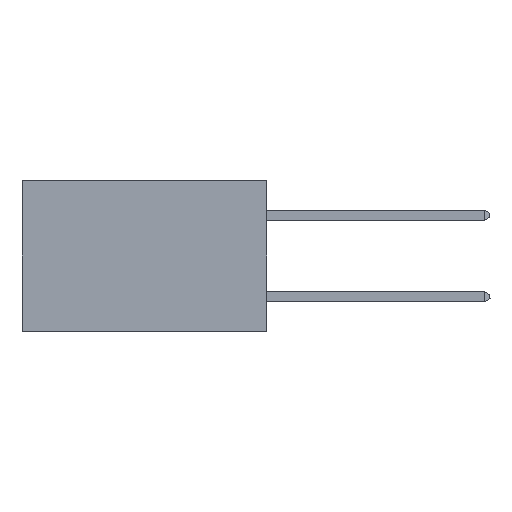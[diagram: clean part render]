
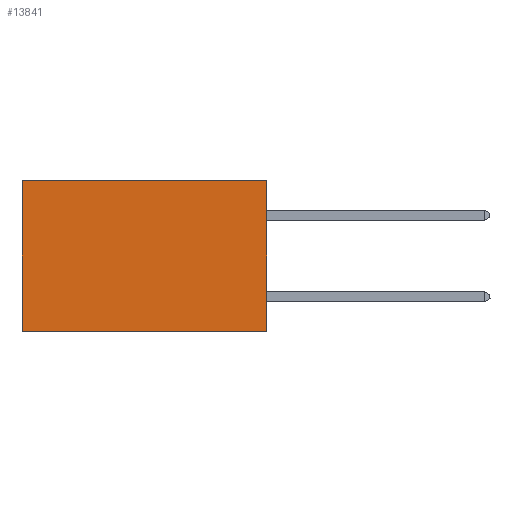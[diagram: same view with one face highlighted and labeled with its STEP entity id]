
A CAD part, left-side view. The second image highlights one B-rep face of the part: STEP entity #13841.
In plain terms, the highlighted planar face has unit normal (-1, 0, 0).
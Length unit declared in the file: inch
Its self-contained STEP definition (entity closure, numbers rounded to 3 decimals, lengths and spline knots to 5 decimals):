
#103 = DIRECTION ( 'NONE',  ( 1., 0., 0. ) ) ;
#491 = VERTEX_POINT ( 'NONE', #4262 ) ;
#1668 = EDGE_CURVE ( 'NONE', #12954, #12230, #16529, .T. ) ;
#2111 = DIRECTION ( 'NONE',  ( 0., 0., -1. ) ) ;
#2417 = EDGE_CURVE ( 'NONE', #12954, #491, #9904, .T. ) ;
#3598 = AXIS2_PLACEMENT_3D ( 'NONE', #10663, #103, #8134 ) ;
#4032 = DIRECTION ( 'NONE',  ( 0., 1., 0. ) ) ;
#4103 = ORIENTED_EDGE ( 'NONE', *, *, #1668, .T. ) ;
#4262 = CARTESIAN_POINT ( 'NONE',  ( 0.2875, 0., -0.37 ) ) ;
#4274 = CARTESIAN_POINT ( 'NONE',  ( 0.2875, 0., 0. ) ) ;
#6805 = PLANE ( 'NONE',  #3598 ) ;
#7149 = VERTEX_POINT ( 'NONE', #11163 ) ;
#7291 = EDGE_CURVE ( 'NONE', #491, #7149, #14238, .T. ) ;
#7792 = CARTESIAN_POINT ( 'NONE',  ( 0.2875, 0., 0. ) ) ;
#8134 = DIRECTION ( 'NONE',  ( 0., 0., -1. ) ) ;
#8281 = EDGE_LOOP ( 'NONE', ( #15273, #16694, #11215, #4103 ) ) ;
#9147 = CARTESIAN_POINT ( 'NONE',  ( 0.2875, 0., 0. ) ) ;
#9434 = DIRECTION ( 'NONE',  ( 0., 0., -1. ) ) ;
#9902 = VECTOR ( 'NONE', #4032, 39.37008 ) ;
#9904 = LINE ( 'NONE', #4274, #15490 ) ;
#10663 = CARTESIAN_POINT ( 'NONE',  ( 0.2875, 0., 0. ) ) ;
#11163 = CARTESIAN_POINT ( 'NONE',  ( 0.2875, 0.6, -0.37 ) ) ;
#11215 = ORIENTED_EDGE ( 'NONE', *, *, #2417, .F. ) ;
#12230 = VERTEX_POINT ( 'NONE', #16249 ) ;
#12257 = CARTESIAN_POINT ( 'NONE',  ( 0.2875, 0., -0.37 ) ) ;
#12954 = VERTEX_POINT ( 'NONE', #9147 ) ;
#13289 = DIRECTION ( 'NONE',  ( 0., 1., 0. ) ) ;
#13841 = ADVANCED_FACE ( 'NONE', ( #15282 ), #6805, .F. ) ;
#13993 = CARTESIAN_POINT ( 'NONE',  ( 0.2875, 0.6, 0. ) ) ;
#14238 = LINE ( 'NONE', #12257, #16549 ) ;
#14711 = EDGE_CURVE ( 'NONE', #12230, #7149, #16672, .T. ) ;
#14991 = VECTOR ( 'NONE', #2111, 39.37008 ) ;
#15273 = ORIENTED_EDGE ( 'NONE', *, *, #14711, .T. ) ;
#15282 = FACE_OUTER_BOUND ( 'NONE', #8281, .T. ) ;
#15490 = VECTOR ( 'NONE', #9434, 39.37008 ) ;
#16249 = CARTESIAN_POINT ( 'NONE',  ( 0.2875, 0.6, 0. ) ) ;
#16529 = LINE ( 'NONE', #7792, #9902 ) ;
#16549 = VECTOR ( 'NONE', #13289, 39.37008 ) ;
#16672 = LINE ( 'NONE', #13993, #14991 ) ;
#16694 = ORIENTED_EDGE ( 'NONE', *, *, #7291, .F. ) ;
